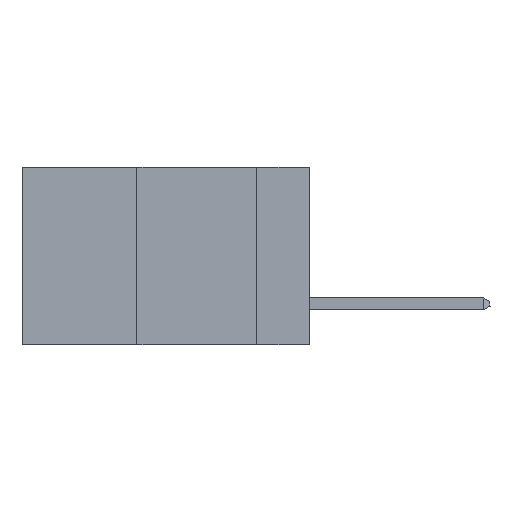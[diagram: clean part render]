
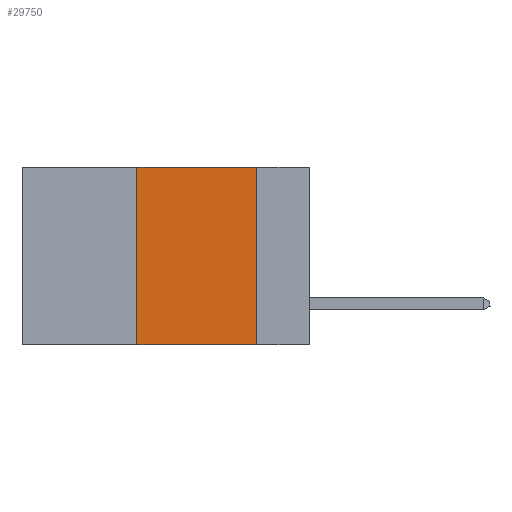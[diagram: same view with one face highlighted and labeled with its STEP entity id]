
A CAD part, left-side view. The second image highlights one B-rep face of the part: STEP entity #29750.
In plain terms, the highlighted planar face has unit normal (-1, 0, 0).
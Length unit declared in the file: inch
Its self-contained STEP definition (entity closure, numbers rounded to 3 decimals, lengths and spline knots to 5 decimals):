
#153 = VERTEX_POINT ( 'NONE', #38201 ) ;
#978 = CARTESIAN_POINT ( 'NONE',  ( 0., 0.11, 0. ) ) ;
#2805 = DIRECTION ( 'NONE',  ( 0., 0., -1. ) ) ;
#2999 = FACE_OUTER_BOUND ( 'NONE', #37745, .T. ) ;
#6020 = DIRECTION ( 'NONE',  ( 0., -1., 0. ) ) ;
#7483 = DIRECTION ( 'NONE',  ( 1., 0., 0. ) ) ;
#7831 = EDGE_CURVE ( 'NONE', #21233, #24088, #33897, .T. ) ;
#8291 = LINE ( 'NONE', #12543, #38858 ) ;
#10548 = EDGE_CURVE ( 'NONE', #24088, #153, #8291, .T. ) ;
#10712 = VECTOR ( 'NONE', #6020, 39.37008 ) ;
#10964 = AXIS2_PLACEMENT_3D ( 'NONE', #40942, #7483, #40637 ) ;
#11850 = CARTESIAN_POINT ( 'NONE',  ( 0., 0.36, 0. ) ) ;
#12225 = ORIENTED_EDGE ( 'NONE', *, *, #22013, .T. ) ;
#12543 = CARTESIAN_POINT ( 'NONE',  ( 0., 0.11, 0. ) ) ;
#15281 = VECTOR ( 'NONE', #16441, 39.37008 ) ;
#16441 = DIRECTION ( 'NONE',  ( 0., -1., 0. ) ) ;
#20382 = CARTESIAN_POINT ( 'NONE',  ( 0., 0.36, -0.37 ) ) ;
#21233 = VERTEX_POINT ( 'NONE', #11850 ) ;
#22013 = EDGE_CURVE ( 'NONE', #27478, #153, #28391, .T. ) ;
#24007 = PLANE ( 'NONE',  #10964 ) ;
#24088 = VERTEX_POINT ( 'NONE', #978 ) ;
#25334 = CARTESIAN_POINT ( 'NONE',  ( 0., 0.6, -0.37 ) ) ;
#27033 = LINE ( 'NONE', #27970, #38410 ) ;
#27478 = VERTEX_POINT ( 'NONE', #20382 ) ;
#27963 = EDGE_CURVE ( 'NONE', #27478, #21233, #27033, .T. ) ;
#27970 = CARTESIAN_POINT ( 'NONE',  ( 0., 0.36, 0. ) ) ;
#28391 = LINE ( 'NONE', #25334, #10712 ) ;
#29061 = ORIENTED_EDGE ( 'NONE', *, *, #10548, .F. ) ;
#29750 = ADVANCED_FACE ( 'NONE', ( #2999 ), #24007, .F. ) ;
#30145 = ORIENTED_EDGE ( 'NONE', *, *, #7831, .F. ) ;
#33897 = LINE ( 'NONE', #41801, #15281 ) ;
#36092 = ORIENTED_EDGE ( 'NONE', *, *, #27963, .F. ) ;
#37745 = EDGE_LOOP ( 'NONE', ( #29061, #30145, #36092, #12225 ) ) ;
#38201 = CARTESIAN_POINT ( 'NONE',  ( 0., 0.11, -0.37 ) ) ;
#38410 = VECTOR ( 'NONE', #40813, 39.37008 ) ;
#38858 = VECTOR ( 'NONE', #2805, 39.37008 ) ;
#40637 = DIRECTION ( 'NONE',  ( 0., 0., -1. ) ) ;
#40813 = DIRECTION ( 'NONE',  ( 0., 0., 1. ) ) ;
#40942 = CARTESIAN_POINT ( 'NONE',  ( 0., 0.6, 0. ) ) ;
#41801 = CARTESIAN_POINT ( 'NONE',  ( 0., 0.6, 0. ) ) ;
